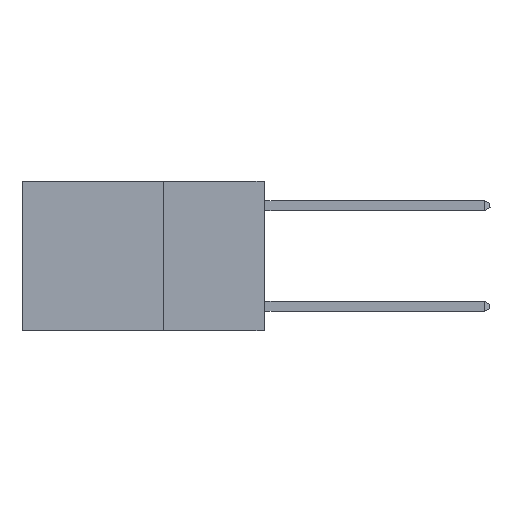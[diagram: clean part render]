
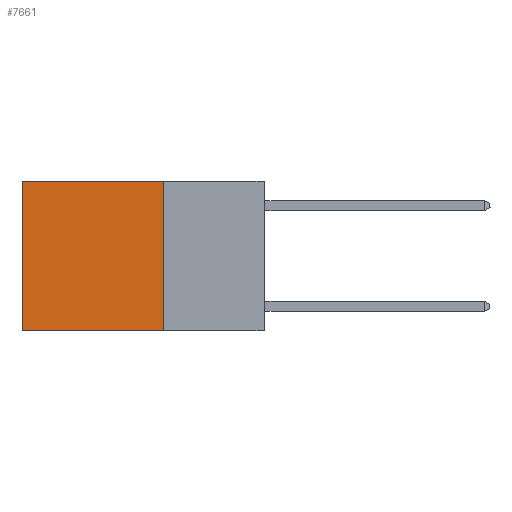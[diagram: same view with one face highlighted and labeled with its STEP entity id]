
A CAD part, left-side view. The second image highlights one B-rep face of the part: STEP entity #7661.
In plain terms, the highlighted planar face has unit normal (-1, 0, 0).
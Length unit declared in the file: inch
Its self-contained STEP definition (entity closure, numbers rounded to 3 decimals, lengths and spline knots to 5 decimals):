
#398 = EDGE_CURVE ( 'NONE', #14736, #8063, #11791, .T. ) ;
#672 = VERTEX_POINT ( 'NONE', #12442 ) ;
#1085 = LINE ( 'NONE', #9266, #3112 ) ;
#1479 = ORIENTED_EDGE ( 'NONE', *, *, #11517, .T. ) ;
#1848 = DIRECTION ( 'NONE',  ( 0., 0., -1. ) ) ;
#3112 = VECTOR ( 'NONE', #11562, 39.37008 ) ;
#4152 = CARTESIAN_POINT ( 'NONE',  ( 0.2625, 0.25, 0. ) ) ;
#4998 = VECTOR ( 'NONE', #10191, 39.37008 ) ;
#5230 = VERTEX_POINT ( 'NONE', #15318 ) ;
#5240 = VECTOR ( 'NONE', #1848, 39.37008 ) ;
#5554 = DIRECTION ( 'NONE',  ( 1., 0., 0. ) ) ;
#5701 = VECTOR ( 'NONE', #15304, 39.37008 ) ;
#5921 = FACE_OUTER_BOUND ( 'NONE', #9784, .T. ) ;
#7368 = LINE ( 'NONE', #12879, #5701 ) ;
#7661 = ADVANCED_FACE ( 'NONE', ( #5921 ), #13666, .F. ) ;
#7953 = CARTESIAN_POINT ( 'NONE',  ( 0.2625, 0.25, 0. ) ) ;
#8063 = VERTEX_POINT ( 'NONE', #11241 ) ;
#8439 = LINE ( 'NONE', #4152, #5240 ) ;
#8867 = CARTESIAN_POINT ( 'NONE',  ( 0.2625, 0.6, 0. ) ) ;
#9103 = CARTESIAN_POINT ( 'NONE',  ( 0.2625, 0.6, 0. ) ) ;
#9211 = EDGE_CURVE ( 'NONE', #672, #5230, #8439, .T. ) ;
#9266 = CARTESIAN_POINT ( 'NONE',  ( 0.2625, 0.25, 0. ) ) ;
#9784 = EDGE_LOOP ( 'NONE', ( #15520, #11876, #14485, #1479 ) ) ;
#10191 = DIRECTION ( 'NONE',  ( 0., 0., -1. ) ) ;
#10958 = AXIS2_PLACEMENT_3D ( 'NONE', #7953, #5554, #14078 ) ;
#11241 = CARTESIAN_POINT ( 'NONE',  ( 0.2625, 0.6, -0.37 ) ) ;
#11517 = EDGE_CURVE ( 'NONE', #672, #14736, #1085, .T. ) ;
#11562 = DIRECTION ( 'NONE',  ( 0., 1., 0. ) ) ;
#11791 = LINE ( 'NONE', #8867, #4998 ) ;
#11876 = ORIENTED_EDGE ( 'NONE', *, *, #13212, .F. ) ;
#12442 = CARTESIAN_POINT ( 'NONE',  ( 0.2625, 0.25, 0. ) ) ;
#12879 = CARTESIAN_POINT ( 'NONE',  ( 0.2625, 0.25, -0.37 ) ) ;
#13212 = EDGE_CURVE ( 'NONE', #5230, #8063, #7368, .T. ) ;
#13666 = PLANE ( 'NONE',  #10958 ) ;
#14078 = DIRECTION ( 'NONE',  ( 0., 0., -1. ) ) ;
#14485 = ORIENTED_EDGE ( 'NONE', *, *, #9211, .F. ) ;
#14736 = VERTEX_POINT ( 'NONE', #9103 ) ;
#15304 = DIRECTION ( 'NONE',  ( 0., 1., 0. ) ) ;
#15318 = CARTESIAN_POINT ( 'NONE',  ( 0.2625, 0.25, -0.37 ) ) ;
#15520 = ORIENTED_EDGE ( 'NONE', *, *, #398, .T. ) ;
